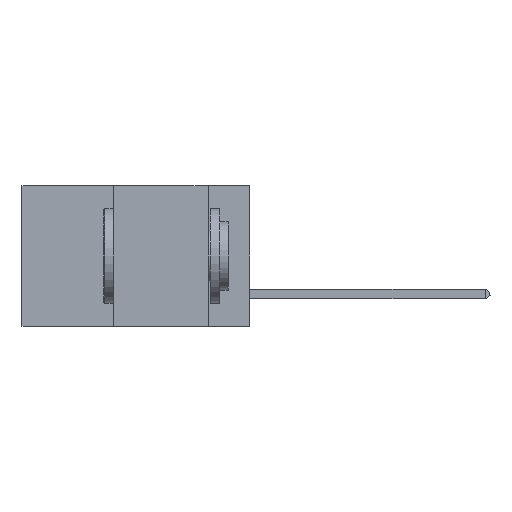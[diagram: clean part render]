
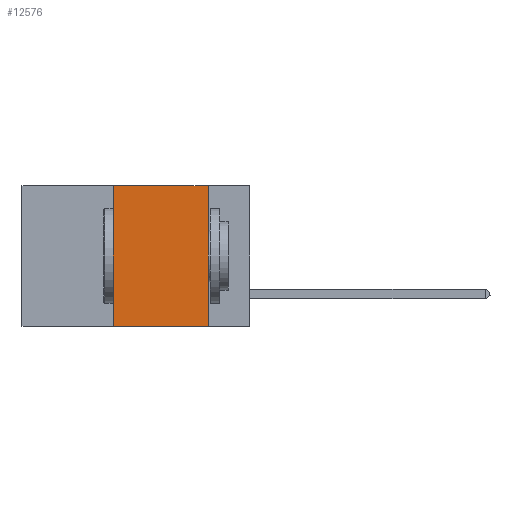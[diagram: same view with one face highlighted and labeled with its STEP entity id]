
A CAD part, left-side view. The second image highlights one B-rep face of the part: STEP entity #12576.
In plain terms, the highlighted planar face has unit normal (-1, 0, 0).
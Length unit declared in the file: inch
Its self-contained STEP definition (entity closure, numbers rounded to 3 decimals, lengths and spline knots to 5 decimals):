
#22 = DIRECTION ( 'NONE',  ( 0., 0., -1. ) ) ;
#108 = ORIENTED_EDGE ( 'NONE', *, *, #8497, .T. ) ;
#424 = EDGE_CURVE ( 'NONE', #3557, #1015, #2024, .T. ) ;
#525 = DIRECTION ( 'NONE',  ( 1., 0., 0. ) ) ;
#1015 = VERTEX_POINT ( 'NONE', #8601 ) ;
#1167 = LINE ( 'NONE', #6205, #2525 ) ;
#1581 = DIRECTION ( 'NONE',  ( 0., 0., -1. ) ) ;
#2012 = FACE_OUTER_BOUND ( 'NONE', #2429, .T. ) ;
#2022 = VECTOR ( 'NONE', #7536, 39.37008 ) ;
#2024 = LINE ( 'NONE', #8729, #12101 ) ;
#2429 = EDGE_LOOP ( 'NONE', ( #3016, #7567, #11048, #108 ) ) ;
#2451 = EDGE_CURVE ( 'NONE', #3562, #3557, #1167, .T. ) ;
#2525 = VECTOR ( 'NONE', #4106, 39.37008 ) ;
#3016 = ORIENTED_EDGE ( 'NONE', *, *, #424, .F. ) ;
#3143 = CARTESIAN_POINT ( 'NONE',  ( 0., 0.6, -0.37 ) ) ;
#3557 = VERTEX_POINT ( 'NONE', #5980 ) ;
#3562 = VERTEX_POINT ( 'NONE', #10922 ) ;
#4106 = DIRECTION ( 'NONE',  ( 0., -1., 0. ) ) ;
#4418 = EDGE_CURVE ( 'NONE', #8079, #3562, #9801, .T. ) ;
#4717 = VECTOR ( 'NONE', #5096, 39.37008 ) ;
#5096 = DIRECTION ( 'NONE',  ( 0., -1., 0. ) ) ;
#5980 = CARTESIAN_POINT ( 'NONE',  ( 0., 0.11, 0. ) ) ;
#6205 = CARTESIAN_POINT ( 'NONE',  ( 0., 0.6, 0. ) ) ;
#6447 = PLANE ( 'NONE',  #8542 ) ;
#7536 = DIRECTION ( 'NONE',  ( 0., 0., 1. ) ) ;
#7567 = ORIENTED_EDGE ( 'NONE', *, *, #2451, .F. ) ;
#8079 = VERTEX_POINT ( 'NONE', #12156 ) ;
#8497 = EDGE_CURVE ( 'NONE', #8079, #1015, #8700, .T. ) ;
#8542 = AXIS2_PLACEMENT_3D ( 'NONE', #10360, #525, #1581 ) ;
#8592 = CARTESIAN_POINT ( 'NONE',  ( 0., 0.36, 0. ) ) ;
#8601 = CARTESIAN_POINT ( 'NONE',  ( 0., 0.11, -0.37 ) ) ;
#8700 = LINE ( 'NONE', #3143, #4717 ) ;
#8729 = CARTESIAN_POINT ( 'NONE',  ( 0., 0.11, 0. ) ) ;
#9801 = LINE ( 'NONE', #8592, #2022 ) ;
#10360 = CARTESIAN_POINT ( 'NONE',  ( 0., 0.6, 0. ) ) ;
#10922 = CARTESIAN_POINT ( 'NONE',  ( 0., 0.36, 0. ) ) ;
#11048 = ORIENTED_EDGE ( 'NONE', *, *, #4418, .F. ) ;
#12101 = VECTOR ( 'NONE', #22, 39.37008 ) ;
#12156 = CARTESIAN_POINT ( 'NONE',  ( 0., 0.36, -0.37 ) ) ;
#12576 = ADVANCED_FACE ( 'NONE', ( #2012 ), #6447, .F. ) ;
